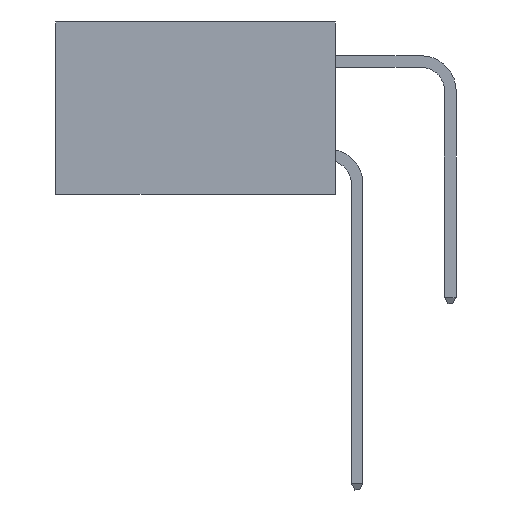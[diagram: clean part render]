
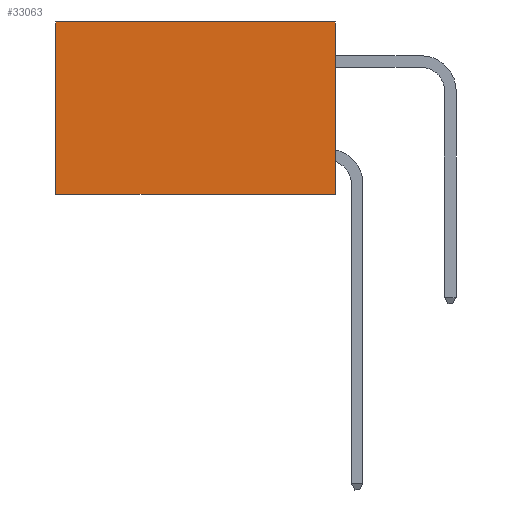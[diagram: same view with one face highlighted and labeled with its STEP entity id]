
A CAD part, left-side view. The second image highlights one B-rep face of the part: STEP entity #33063.
In plain terms, the highlighted planar face has unit normal (-1, 0, 0).
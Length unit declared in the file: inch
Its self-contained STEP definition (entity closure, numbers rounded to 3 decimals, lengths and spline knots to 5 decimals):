
#338 = EDGE_CURVE ( 'NONE', #37876, #5239, #15591, .T. ) ;
#657 = CARTESIAN_POINT ( 'NONE',  ( 0.2875, 0.6, -0.37 ) ) ;
#1157 = VECTOR ( 'NONE', #21787, 39.37008 ) ;
#5239 = VERTEX_POINT ( 'NONE', #657 ) ;
#5686 = CARTESIAN_POINT ( 'NONE',  ( 0.2875, 0.6, 0. ) ) ;
#9780 = FACE_OUTER_BOUND ( 'NONE', #34688, .T. ) ;
#10280 = VERTEX_POINT ( 'NONE', #30442 ) ;
#11366 = CARTESIAN_POINT ( 'NONE',  ( 0.2875, 0., -0.37 ) ) ;
#11375 = VECTOR ( 'NONE', #19187, 39.37008 ) ;
#15591 = LINE ( 'NONE', #5686, #11375 ) ;
#16715 = ORIENTED_EDGE ( 'NONE', *, *, #19459, .F. ) ;
#17051 = AXIS2_PLACEMENT_3D ( 'NONE', #24044, #27725, #17615 ) ;
#17615 = DIRECTION ( 'NONE',  ( 0., 0., -1. ) ) ;
#17928 = EDGE_CURVE ( 'NONE', #10280, #37876, #19102, .T. ) ;
#18279 = VERTEX_POINT ( 'NONE', #41831 ) ;
#18573 = CARTESIAN_POINT ( 'NONE',  ( 0.2875, 0., 0. ) ) ;
#19102 = LINE ( 'NONE', #18573, #1157 ) ;
#19187 = DIRECTION ( 'NONE',  ( 0., 0., -1. ) ) ;
#19274 = ORIENTED_EDGE ( 'NONE', *, *, #17928, .T. ) ;
#19459 = EDGE_CURVE ( 'NONE', #10280, #18279, #23115, .T. ) ;
#19618 = VECTOR ( 'NONE', #28668, 39.37008 ) ;
#20678 = CARTESIAN_POINT ( 'NONE',  ( 0.2875, 0.6, 0. ) ) ;
#21787 = DIRECTION ( 'NONE',  ( 0., 1., 0. ) ) ;
#22219 = LINE ( 'NONE', #11366, #19618 ) ;
#23115 = LINE ( 'NONE', #32197, #28389 ) ;
#23662 = ORIENTED_EDGE ( 'NONE', *, *, #28635, .F. ) ;
#24044 = CARTESIAN_POINT ( 'NONE',  ( 0.2875, 0., 0. ) ) ;
#26043 = ORIENTED_EDGE ( 'NONE', *, *, #338, .T. ) ;
#27725 = DIRECTION ( 'NONE',  ( 1., 0., 0. ) ) ;
#28389 = VECTOR ( 'NONE', #42366, 39.37008 ) ;
#28635 = EDGE_CURVE ( 'NONE', #18279, #5239, #22219, .T. ) ;
#28668 = DIRECTION ( 'NONE',  ( 0., 1., 0. ) ) ;
#30442 = CARTESIAN_POINT ( 'NONE',  ( 0.2875, 0., 0. ) ) ;
#32197 = CARTESIAN_POINT ( 'NONE',  ( 0.2875, 0., 0. ) ) ;
#33063 = ADVANCED_FACE ( 'NONE', ( #9780 ), #34175, .F. ) ;
#34175 = PLANE ( 'NONE',  #17051 ) ;
#34688 = EDGE_LOOP ( 'NONE', ( #26043, #23662, #16715, #19274 ) ) ;
#37876 = VERTEX_POINT ( 'NONE', #20678 ) ;
#41831 = CARTESIAN_POINT ( 'NONE',  ( 0.2875, 0., -0.37 ) ) ;
#42366 = DIRECTION ( 'NONE',  ( 0., 0., -1. ) ) ;
